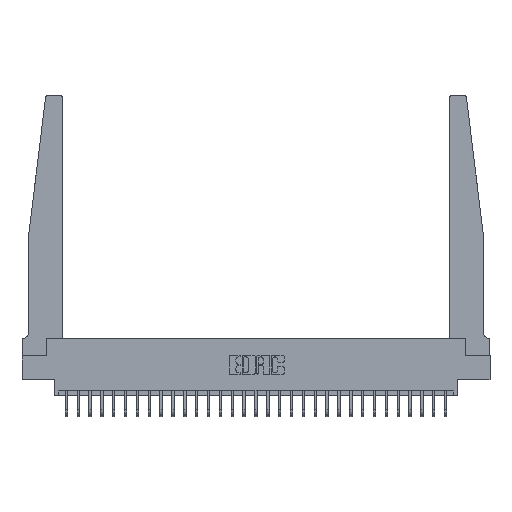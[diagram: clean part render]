
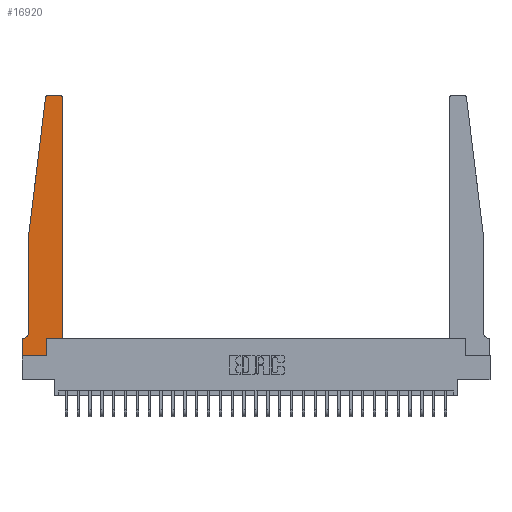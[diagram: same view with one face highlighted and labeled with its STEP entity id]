
A CAD part, top view. The second image highlights one B-rep face of the part: STEP entity #16920.
In plain terms, the highlighted planar face has unit normal (0, 0, 1).
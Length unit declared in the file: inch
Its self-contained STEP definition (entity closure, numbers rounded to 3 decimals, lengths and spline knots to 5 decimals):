
#11 = DIRECTION ( 'NONE',  ( 0., 0., -1. ) ) ;
#36 = CIRCLE ( 'NONE', #1274, 0.03 ) ;
#423 = ORIENTED_EDGE ( 'NONE', *, *, #6511, .T. ) ;
#437 = VECTOR ( 'NONE', #26122, 39.37008 ) ;
#606 = CARTESIAN_POINT ( 'NONE',  ( 0., 0.1875, 0.37 ) ) ;
#1274 = AXIS2_PLACEMENT_3D ( 'NONE', #19381, #26707, #26906 ) ;
#1305 = VECTOR ( 'NONE', #26702, 39.37008 ) ;
#1516 = CARTESIAN_POINT ( 'NONE',  ( 0.2605, 0., 0.37 ) ) ;
#1582 = CARTESIAN_POINT ( 'NONE',  ( 0.27653, 2.75, 0.37 ) ) ;
#2045 = EDGE_CURVE ( 'NONE', #7397, #10172, #4815, .T. ) ;
#2660 = VECTOR ( 'NONE', #18535, 39.37008 ) ;
#3001 = CARTESIAN_POINT ( 'NONE',  ( 0., 0., 0.37 ) ) ;
#3043 = ORIENTED_EDGE ( 'NONE', *, *, #10358, .T. ) ;
#3306 = VECTOR ( 'NONE', #12401, 39.37008 ) ;
#3359 = ORIENTED_EDGE ( 'NONE', *, *, #22514, .T. ) ;
#3510 = EDGE_CURVE ( 'NONE', #15471, #19813, #3650, .T. ) ;
#3569 = EDGE_CURVE ( 'NONE', #11036, #4610, #16774, .T. ) ;
#3650 = LINE ( 'NONE', #14397, #3306 ) ;
#3972 = EDGE_LOOP ( 'NONE', ( #423, #3359, #9991, #3043, #4783, #20950, #27858, #5952, #28776, #14268, #24199, #18429 ) ) ;
#4036 = CIRCLE ( 'NONE', #10616, 0.03 ) ;
#4551 = CARTESIAN_POINT ( 'NONE',  ( 0.25, 2.75, 0.37 ) ) ;
#4610 = VERTEX_POINT ( 'NONE', #13124 ) ;
#4742 = DIRECTION ( 'NONE',  ( -1., 0., 0. ) ) ;
#4783 = ORIENTED_EDGE ( 'NONE', *, *, #26714, .T. ) ;
#4797 = LINE ( 'NONE', #24010, #2660 ) ;
#4815 = LINE ( 'NONE', #4828, #16490 ) ;
#4828 = CARTESIAN_POINT ( 'NONE',  ( 0.425, 0.18, 0.37 ) ) ;
#5196 = CARTESIAN_POINT ( 'NONE',  ( 0.425, 2.72, 0.37 ) ) ;
#5952 = ORIENTED_EDGE ( 'NONE', *, *, #11446, .T. ) ;
#6170 = CARTESIAN_POINT ( 'NONE',  ( 0.065, 1.25, 0.37 ) ) ;
#6400 = DIRECTION ( 'NONE',  ( 0., 0., 1. ) ) ;
#6511 = EDGE_CURVE ( 'NONE', #27384, #11557, #26594, .T. ) ;
#6596 = VECTOR ( 'NONE', #14457, 39.37008 ) ;
#6709 = CARTESIAN_POINT ( 'NONE',  ( 0.2605, 0.18, 0.37 ) ) ;
#7370 = CARTESIAN_POINT ( 'NONE',  ( 0.425, 0.18, 0.37 ) ) ;
#7397 = VERTEX_POINT ( 'NONE', #6709 ) ;
#7713 = EDGE_CURVE ( 'NONE', #18541, #27384, #36, .T. ) ;
#8674 = FACE_OUTER_BOUND ( 'NONE', #3972, .T. ) ;
#9139 = DIRECTION ( 'NONE',  ( 1., 0., 0. ) ) ;
#9569 = VECTOR ( 'NONE', #4742, 39.37008 ) ;
#9991 = ORIENTED_EDGE ( 'NONE', *, *, #3569, .T. ) ;
#10172 = VERTEX_POINT ( 'NONE', #7370 ) ;
#10358 = EDGE_CURVE ( 'NONE', #4610, #24301, #18352, .T. ) ;
#10616 = AXIS2_PLACEMENT_3D ( 'NONE', #20367, #6400, #9139 ) ;
#11036 = VERTEX_POINT ( 'NONE', #13175 ) ;
#11446 = EDGE_CURVE ( 'NONE', #23266, #26365, #17222, .T. ) ;
#11544 = DIRECTION ( 'NONE',  ( 1., 0., 0. ) ) ;
#11557 = VERTEX_POINT ( 'NONE', #1582 ) ;
#12030 = EDGE_CURVE ( 'NONE', #10172, #18541, #14713, .T. ) ;
#12401 = DIRECTION ( 'NONE',  ( -1., 0., 0. ) ) ;
#13124 = CARTESIAN_POINT ( 'NONE',  ( 0.065, 1.25, 0.37 ) ) ;
#13175 = CARTESIAN_POINT ( 'NONE',  ( 0.24675, 2.72367, 0.37 ) ) ;
#13326 = AXIS2_PLACEMENT_3D ( 'NONE', #13582, #11, #15895 ) ;
#13388 = DIRECTION ( 'NONE',  ( 0., 1., 0. ) ) ;
#13582 = CARTESIAN_POINT ( 'NONE',  ( 0.015, 0.2375, 0.37 ) ) ;
#13834 = CARTESIAN_POINT ( 'NONE',  ( 0.395, 2.75, 0.37 ) ) ;
#14268 = ORIENTED_EDGE ( 'NONE', *, *, #2045, .T. ) ;
#14397 = CARTESIAN_POINT ( 'NONE',  ( 0.065, 0.1875, 0.37 ) ) ;
#14457 = DIRECTION ( 'NONE',  ( 1., 0., 0. ) ) ;
#14679 = CARTESIAN_POINT ( 'NONE',  ( 0.065, 1.25, 0.37 ) ) ;
#14713 = LINE ( 'NONE', #24769, #20101 ) ;
#15067 = CARTESIAN_POINT ( 'NONE',  ( 0., 0., 0.37 ) ) ;
#15471 = VERTEX_POINT ( 'NONE', #19547 ) ;
#15895 = DIRECTION ( 'NONE',  ( -1., 0., 0. ) ) ;
#16090 = DIRECTION ( 'NONE',  ( 0., 0., 1. ) ) ;
#16490 = VECTOR ( 'NONE', #11544, 39.37008 ) ;
#16774 = LINE ( 'NONE', #14679, #437 ) ;
#16840 = EDGE_CURVE ( 'NONE', #26365, #7397, #4797, .T. ) ;
#16920 = ADVANCED_FACE ( 'NONE', ( #8674 ), #24953, .T. ) ;
#17222 = LINE ( 'NONE', #3001, #6596 ) ;
#18352 = LINE ( 'NONE', #6170, #1305 ) ;
#18377 = DIRECTION ( 'NONE',  ( 1., 0., 0. ) ) ;
#18429 = ORIENTED_EDGE ( 'NONE', *, *, #7713, .T. ) ;
#18535 = DIRECTION ( 'NONE',  ( 0., 1., 0. ) ) ;
#18541 = VERTEX_POINT ( 'NONE', #5196 ) ;
#19381 = CARTESIAN_POINT ( 'NONE',  ( 0.395, 2.72, 0.37 ) ) ;
#19547 = CARTESIAN_POINT ( 'NONE',  ( 0.015, 0.1875, 0.37 ) ) ;
#19671 = DIRECTION ( 'NONE',  ( 0., -1., 0. ) ) ;
#19813 = VERTEX_POINT ( 'NONE', #606 ) ;
#20079 = CARTESIAN_POINT ( 'NONE',  ( 0.065, 0.2375, 0.37 ) ) ;
#20101 = VECTOR ( 'NONE', #13388, 39.37008 ) ;
#20367 = CARTESIAN_POINT ( 'NONE',  ( 0.27653, 2.72, 0.37 ) ) ;
#20482 = CIRCLE ( 'NONE', #13326, 0.05 ) ;
#20806 = CARTESIAN_POINT ( 'NONE',  ( 0., 0., 0.37 ) ) ;
#20950 = ORIENTED_EDGE ( 'NONE', *, *, #3510, .T. ) ;
#21042 = EDGE_CURVE ( 'NONE', #19813, #23266, #22197, .T. ) ;
#22197 = LINE ( 'NONE', #15067, #27481 ) ;
#22514 = EDGE_CURVE ( 'NONE', #11557, #11036, #4036, .T. ) ;
#23266 = VERTEX_POINT ( 'NONE', #20806 ) ;
#24010 = CARTESIAN_POINT ( 'NONE',  ( 0.2605, 0.18, 0.37 ) ) ;
#24199 = ORIENTED_EDGE ( 'NONE', *, *, #12030, .T. ) ;
#24301 = VERTEX_POINT ( 'NONE', #20079 ) ;
#24769 = CARTESIAN_POINT ( 'NONE',  ( 0.425, 0.18, 0.37 ) ) ;
#24953 = PLANE ( 'NONE',  #27311 ) ;
#25135 = CARTESIAN_POINT ( 'NONE',  ( 0., 0.1875, 0.37 ) ) ;
#26122 = DIRECTION ( 'NONE',  ( -0.122, -0.992, 0. ) ) ;
#26365 = VERTEX_POINT ( 'NONE', #1516 ) ;
#26594 = LINE ( 'NONE', #4551, #9569 ) ;
#26702 = DIRECTION ( 'NONE',  ( 0., -1., 0. ) ) ;
#26707 = DIRECTION ( 'NONE',  ( 0., 0., 1. ) ) ;
#26714 = EDGE_CURVE ( 'NONE', #24301, #15471, #20482, .T. ) ;
#26906 = DIRECTION ( 'NONE',  ( 1., 0., 0. ) ) ;
#27311 = AXIS2_PLACEMENT_3D ( 'NONE', #25135, #16090, #18377 ) ;
#27384 = VERTEX_POINT ( 'NONE', #13834 ) ;
#27481 = VECTOR ( 'NONE', #19671, 39.37008 ) ;
#27858 = ORIENTED_EDGE ( 'NONE', *, *, #21042, .T. ) ;
#28776 = ORIENTED_EDGE ( 'NONE', *, *, #16840, .T. ) ;
